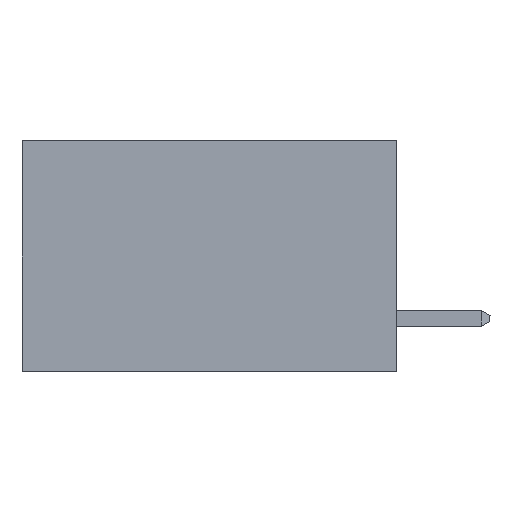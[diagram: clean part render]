
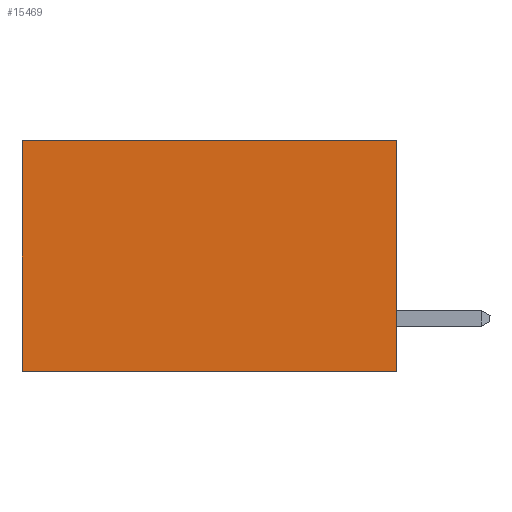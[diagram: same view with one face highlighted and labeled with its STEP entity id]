
A CAD part, left-side view. The second image highlights one B-rep face of the part: STEP entity #15469.
In plain terms, the highlighted planar face has unit normal (-1, 0, 0).
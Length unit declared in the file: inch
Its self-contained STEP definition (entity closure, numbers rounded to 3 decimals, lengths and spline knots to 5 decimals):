
#441 = CARTESIAN_POINT ( 'NONE',  ( 0.2615, 0., -0.37 ) ) ;
#870 = CARTESIAN_POINT ( 'NONE',  ( 0.2615, 0.6, -0.37 ) ) ;
#1240 = DIRECTION ( 'NONE',  ( 0., 0., -1. ) ) ;
#2419 = CARTESIAN_POINT ( 'NONE',  ( 0.2615, 0., 0. ) ) ;
#2428 = ORIENTED_EDGE ( 'NONE', *, *, #19884, .T. ) ;
#2991 = DIRECTION ( 'NONE',  ( 0., 0., -1. ) ) ;
#3248 = CARTESIAN_POINT ( 'NONE',  ( 0.2615, 0., -0.37 ) ) ;
#3647 = DIRECTION ( 'NONE',  ( 0., 1., 0. ) ) ;
#4033 = LINE ( 'NONE', #3248, #16687 ) ;
#4307 = VERTEX_POINT ( 'NONE', #18889 ) ;
#4362 = VECTOR ( 'NONE', #12384, 39.37008 ) ;
#6200 = EDGE_CURVE ( 'NONE', #12417, #8440, #20107, .T. ) ;
#7459 = ORIENTED_EDGE ( 'NONE', *, *, #8751, .F. ) ;
#8440 = VERTEX_POINT ( 'NONE', #13468 ) ;
#8690 = CARTESIAN_POINT ( 'NONE',  ( 0.2615, 0.6, 0. ) ) ;
#8751 = EDGE_CURVE ( 'NONE', #14299, #4307, #4033, .T. ) ;
#9377 = ORIENTED_EDGE ( 'NONE', *, *, #17949, .F. ) ;
#9565 = CARTESIAN_POINT ( 'NONE',  ( 0.2615, 0., -0.37 ) ) ;
#9742 = AXIS2_PLACEMENT_3D ( 'NONE', #9565, #20796, #11241 ) ;
#9781 = EDGE_LOOP ( 'NONE', ( #18028, #9377, #7459, #2428 ) ) ;
#10300 = CARTESIAN_POINT ( 'NONE',  ( 0.2615, 0., 0. ) ) ;
#10754 = VECTOR ( 'NONE', #3647, 39.37008 ) ;
#11070 = VECTOR ( 'NONE', #1240, 39.37008 ) ;
#11241 = DIRECTION ( 'NONE',  ( 0., 0., -1. ) ) ;
#11263 = LINE ( 'NONE', #441, #10754 ) ;
#12384 = DIRECTION ( 'NONE',  ( 0., 1., 0. ) ) ;
#12417 = VERTEX_POINT ( 'NONE', #8690 ) ;
#12620 = FACE_OUTER_BOUND ( 'NONE', #9781, .T. ) ;
#12806 = PLANE ( 'NONE',  #9742 ) ;
#13468 = CARTESIAN_POINT ( 'NONE',  ( 0.2615, 0.6, -0.37 ) ) ;
#14299 = VERTEX_POINT ( 'NONE', #10300 ) ;
#15469 = ADVANCED_FACE ( 'NONE', ( #12620 ), #12806, .F. ) ;
#16687 = VECTOR ( 'NONE', #2991, 39.37008 ) ;
#17507 = LINE ( 'NONE', #2419, #4362 ) ;
#17949 = EDGE_CURVE ( 'NONE', #4307, #8440, #11263, .T. ) ;
#18028 = ORIENTED_EDGE ( 'NONE', *, *, #6200, .T. ) ;
#18889 = CARTESIAN_POINT ( 'NONE',  ( 0.2615, 0., -0.37 ) ) ;
#19884 = EDGE_CURVE ( 'NONE', #14299, #12417, #17507, .T. ) ;
#20107 = LINE ( 'NONE', #870, #11070 ) ;
#20796 = DIRECTION ( 'NONE',  ( 1., 0., 0. ) ) ;
